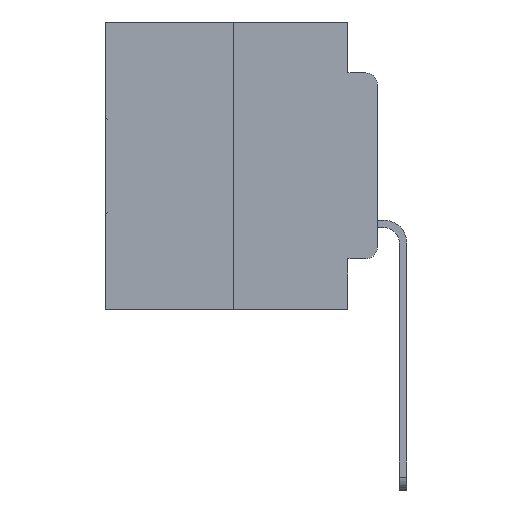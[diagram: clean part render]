
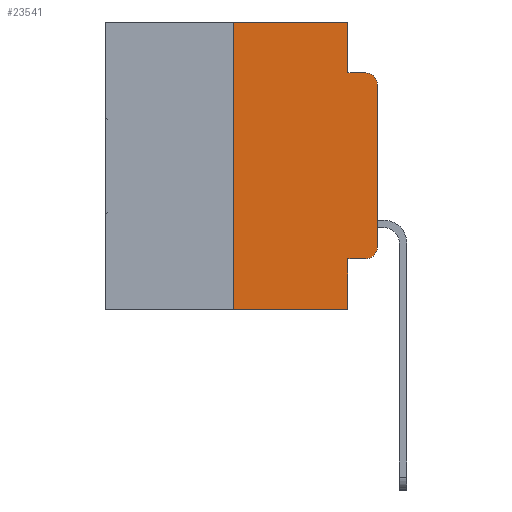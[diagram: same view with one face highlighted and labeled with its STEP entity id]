
A CAD part, left-side view. The second image highlights one B-rep face of the part: STEP entity #23541.
In plain terms, the highlighted planar face has unit normal (-1, 0, 0).
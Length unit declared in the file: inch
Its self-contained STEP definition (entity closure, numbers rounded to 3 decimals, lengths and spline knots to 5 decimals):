
#490 = CIRCLE ( 'NONE', #12257, 0.02 ) ;
#557 = VECTOR ( 'NONE', #3349, 39.37008 ) ;
#781 = EDGE_CURVE ( 'NONE', #11528, #10835, #6993, .T. ) ;
#1464 = VERTEX_POINT ( 'NONE', #2788 ) ;
#1592 = DIRECTION ( 'NONE',  ( 0., 0., 1. ) ) ;
#2000 = VECTOR ( 'NONE', #1592, 39.37008 ) ;
#2626 = ORIENTED_EDGE ( 'NONE', *, *, #6603, .T. ) ;
#2788 = CARTESIAN_POINT ( 'NONE',  ( 0., 0.051, -0.4115 ) ) ;
#2795 = AXIS2_PLACEMENT_3D ( 'NONE', #12169, #27947, #14480 ) ;
#3225 = DIRECTION ( 'NONE',  ( 0., -1., 0. ) ) ;
#3349 = DIRECTION ( 'NONE',  ( 0., 0., -1. ) ) ;
#4107 = LINE ( 'NONE', #8927, #16377 ) ;
#4229 = ORIENTED_EDGE ( 'NONE', *, *, #16619, .F. ) ;
#4811 = LINE ( 'NONE', #12130, #28964 ) ;
#5278 = LINE ( 'NONE', #11181, #16061 ) ;
#5478 = CARTESIAN_POINT ( 'NONE',  ( 0., 0.051, 0. ) ) ;
#6603 = EDGE_CURVE ( 'NONE', #1464, #7990, #4811, .T. ) ;
#6852 = ORIENTED_EDGE ( 'NONE', *, *, #9206, .F. ) ;
#6993 = LINE ( 'NONE', #5478, #557 ) ;
#7716 = CARTESIAN_POINT ( 'NONE',  ( 0., 0.051, -0.0885 ) ) ;
#7981 = CARTESIAN_POINT ( 'NONE',  ( 0., 0.02, -0.1085 ) ) ;
#7990 = VERTEX_POINT ( 'NONE', #8056 ) ;
#8056 = CARTESIAN_POINT ( 'NONE',  ( 0., 0.02, -0.4115 ) ) ;
#8197 = PLANE ( 'NONE',  #16956 ) ;
#8291 = DIRECTION ( 'NONE',  ( 0., -1., 0. ) ) ;
#8842 = CIRCLE ( 'NONE', #2795, 0.02 ) ;
#8927 = CARTESIAN_POINT ( 'NONE',  ( 0., 0.051, 0. ) ) ;
#9206 = EDGE_CURVE ( 'NONE', #28842, #11528, #29185, .T. ) ;
#9948 = VERTEX_POINT ( 'NONE', #13664 ) ;
#10284 = DIRECTION ( 'NONE',  ( 0., 0., -1. ) ) ;
#10396 = EDGE_LOOP ( 'NONE', ( #14178, #12556, #4229, #15816, #6852, #18227, #23565, #18286, #2626, #21814 ) ) ;
#10572 = CARTESIAN_POINT ( 'NONE',  ( 0., 0.25, 0. ) ) ;
#10595 = CARTESIAN_POINT ( 'NONE',  ( 0., 0.473, 0. ) ) ;
#10835 = VERTEX_POINT ( 'NONE', #7716 ) ;
#11181 = CARTESIAN_POINT ( 'NONE',  ( 0., 0.473, -0.5 ) ) ;
#11528 = VERTEX_POINT ( 'NONE', #16648 ) ;
#12130 = CARTESIAN_POINT ( 'NONE',  ( 0., 0.051, -0.4115 ) ) ;
#12169 = CARTESIAN_POINT ( 'NONE',  ( 0., 0.02, -0.3915 ) ) ;
#12172 = VERTEX_POINT ( 'NONE', #12197 ) ;
#12197 = CARTESIAN_POINT ( 'NONE',  ( 0., 0., -0.1085 ) ) ;
#12226 = CARTESIAN_POINT ( 'NONE',  ( 0., 0., -0.3915 ) ) ;
#12257 = AXIS2_PLACEMENT_3D ( 'NONE', #7981, #23882, #10284 ) ;
#12556 = ORIENTED_EDGE ( 'NONE', *, *, #18918, .T. ) ;
#12800 = CARTESIAN_POINT ( 'NONE',  ( 0., 0.473, 0. ) ) ;
#13153 = VECTOR ( 'NONE', #21809, 39.37008 ) ;
#13289 = CARTESIAN_POINT ( 'NONE',  ( 0., 0.25, 0. ) ) ;
#13463 = VERTEX_POINT ( 'NONE', #12226 ) ;
#13664 = CARTESIAN_POINT ( 'NONE',  ( 0., 0.051, -0.5 ) ) ;
#14178 = ORIENTED_EDGE ( 'NONE', *, *, #25448, .T. ) ;
#14480 = DIRECTION ( 'NONE',  ( 0., 0., -1. ) ) ;
#15093 = DIRECTION ( 'NONE',  ( 0., 0., -1. ) ) ;
#15199 = CARTESIAN_POINT ( 'NONE',  ( 0., 0.02, -0.0885 ) ) ;
#15267 = EDGE_CURVE ( 'NONE', #7990, #13463, #8842, .T. ) ;
#15655 = VERTEX_POINT ( 'NONE', #26947 ) ;
#15816 = ORIENTED_EDGE ( 'NONE', *, *, #781, .F. ) ;
#16059 = CARTESIAN_POINT ( 'NONE',  ( 0., 0., 0. ) ) ;
#16061 = VECTOR ( 'NONE', #29212, 39.37008 ) ;
#16377 = VECTOR ( 'NONE', #27020, 39.37008 ) ;
#16560 = VECTOR ( 'NONE', #8291, 39.37008 ) ;
#16619 = EDGE_CURVE ( 'NONE', #10835, #23577, #27572, .T. ) ;
#16648 = CARTESIAN_POINT ( 'NONE',  ( 0., 0.051, 0. ) ) ;
#16956 = AXIS2_PLACEMENT_3D ( 'NONE', #12800, #28564, #15093 ) ;
#17018 = CARTESIAN_POINT ( 'NONE',  ( 0., 0.051, -0.0885 ) ) ;
#18227 = ORIENTED_EDGE ( 'NONE', *, *, #27737, .F. ) ;
#18286 = ORIENTED_EDGE ( 'NONE', *, *, #22153, .F. ) ;
#18918 = EDGE_CURVE ( 'NONE', #12172, #23577, #490, .T. ) ;
#19241 = LINE ( 'NONE', #10572, #13153 ) ;
#19550 = FACE_OUTER_BOUND ( 'NONE', #10396, .T. ) ;
#19786 = LINE ( 'NONE', #16059, #2000 ) ;
#21493 = EDGE_CURVE ( 'NONE', #15655, #9948, #5278, .T. ) ;
#21651 = VECTOR ( 'NONE', #3225, 39.37008 ) ;
#21809 = DIRECTION ( 'NONE',  ( 0., 0., 1. ) ) ;
#21814 = ORIENTED_EDGE ( 'NONE', *, *, #15267, .T. ) ;
#22153 = EDGE_CURVE ( 'NONE', #1464, #9948, #4107, .T. ) ;
#23541 = ADVANCED_FACE ( 'NONE', ( #19550 ), #8197, .F. ) ;
#23565 = ORIENTED_EDGE ( 'NONE', *, *, #21493, .T. ) ;
#23577 = VERTEX_POINT ( 'NONE', #15199 ) ;
#23882 = DIRECTION ( 'NONE',  ( -1., 0., 0. ) ) ;
#25448 = EDGE_CURVE ( 'NONE', #13463, #12172, #19786, .T. ) ;
#26947 = CARTESIAN_POINT ( 'NONE',  ( 0., 0.25, -0.5 ) ) ;
#27020 = DIRECTION ( 'NONE',  ( 0., 0., -1. ) ) ;
#27572 = LINE ( 'NONE', #17018, #21651 ) ;
#27737 = EDGE_CURVE ( 'NONE', #15655, #28842, #19241, .T. ) ;
#27899 = DIRECTION ( 'NONE',  ( 0., -1., 0. ) ) ;
#27947 = DIRECTION ( 'NONE',  ( -1., 0., 0. ) ) ;
#28564 = DIRECTION ( 'NONE',  ( 1., 0., 0. ) ) ;
#28842 = VERTEX_POINT ( 'NONE', #13289 ) ;
#28964 = VECTOR ( 'NONE', #27899, 39.37008 ) ;
#29185 = LINE ( 'NONE', #10595, #16560 ) ;
#29212 = DIRECTION ( 'NONE',  ( 0., -1., 0. ) ) ;
